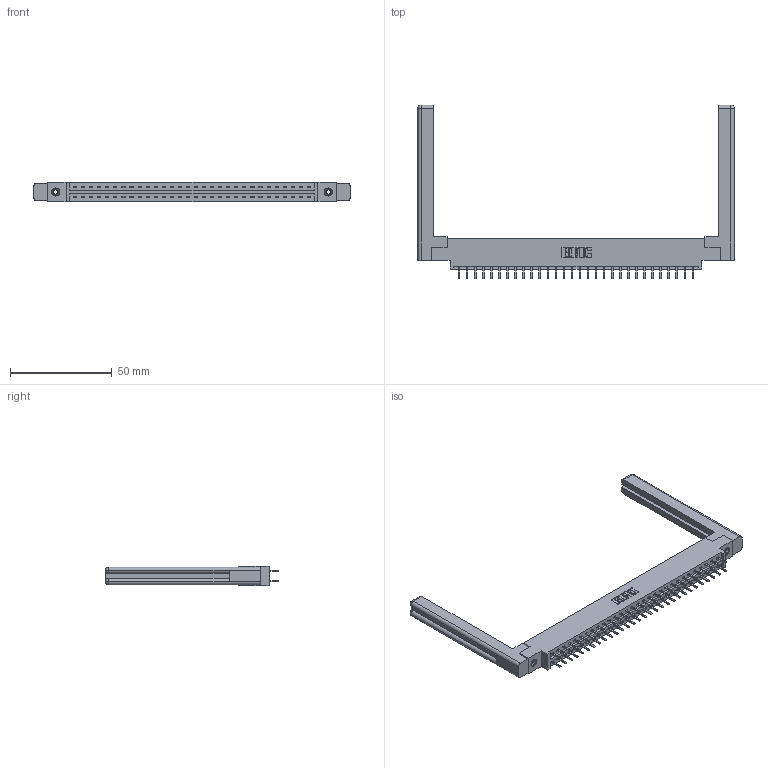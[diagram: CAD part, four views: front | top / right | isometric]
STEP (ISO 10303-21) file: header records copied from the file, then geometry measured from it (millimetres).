
FILE_DESCRIPTION (( 'STEP AP203' ), '1' );
FILE_NAME ('337-060-520-858.STEP', '2019-10-11T21:23:07', ( '' ), ( '' ), 'SwSTEP 2.0', 'SolidWorks 2016', '' );
FILE_SCHEMA (( 'CONFIG_CONTROL_DESIGN' ));
Length unit declared in the file: inch
Products named in the file (5): 345-250-001_345-250-001-102; 307-220-058; 337 Part_0.170 Offset - 0.156 Dia-TI; 345-292-001_345-293-120; 337-060-520-858
Assembly tree (65 placements, depth 2):
  337-060-520-858
    337 Part_0.170 Offset - 0.156 Dia-TI
    345-292-001_345-293-120  x60
    345-250-001_345-250-001-102  x2
    307-220-058  x2
Bounding box: 155.5 x 85.43 x 9.4 mm (x, y, z)
Volume: 23226.4 mm3; surface area: 23145.9 mm2
Topology: 65 solids, 65 shells, 3740 faces, 10817 edges, 7038 vertices
Faces by surface type: plane 2558, cylinder 1158, cone 12, torus 12
Entity records: 27692 total; most frequent: CARTESIAN_POINT 4697, ORIENTED_EDGE 4560, DIRECTION 4020, EDGE_CURVE 2280, LINE 2100, VECTOR 2100, VERTEX_POINT 1510, AXIS2_PLACEMENT_3D 960
